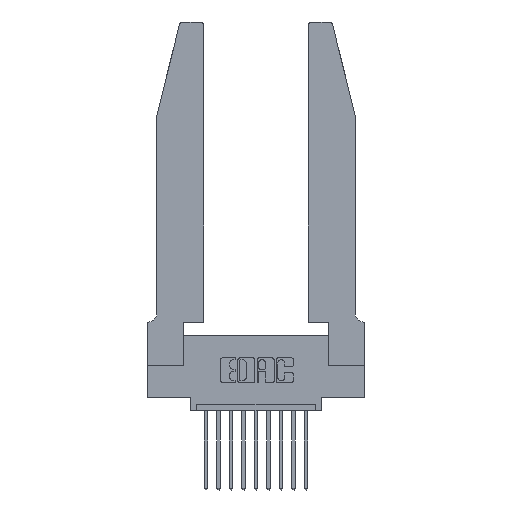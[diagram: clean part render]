
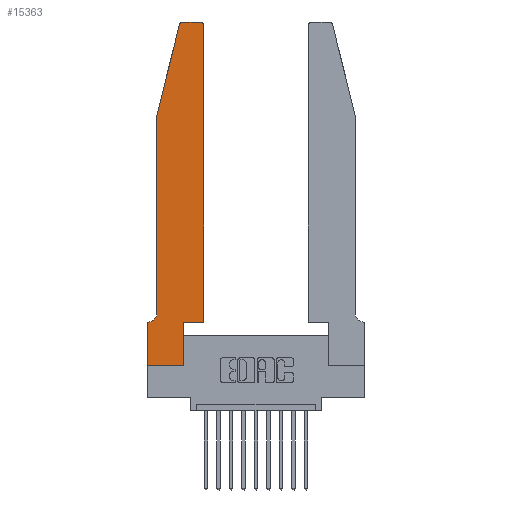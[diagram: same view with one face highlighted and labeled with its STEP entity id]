
A CAD part, top view. The second image highlights one B-rep face of the part: STEP entity #15363.
In plain terms, the highlighted planar face has unit normal (0, 0, 1).
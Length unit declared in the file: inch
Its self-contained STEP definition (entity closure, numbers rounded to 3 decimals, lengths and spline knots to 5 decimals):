
#105 = VECTOR ( 'NONE', #4149, 39.37008 ) ;
#150 = CARTESIAN_POINT ( 'NONE',  ( 0.0755, 0.35, 0.37 ) ) ;
#258 = CARTESIAN_POINT ( 'NONE',  ( 0.2865, 0.35, 0.37 ) ) ;
#534 = FACE_OUTER_BOUND ( 'NONE', #7248, .T. ) ;
#612 = AXIS2_PLACEMENT_3D ( 'NONE', #5074, #13812, #15102 ) ;
#691 = EDGE_CURVE ( 'NONE', #771, #15795, #4961, .T. ) ;
#771 = VERTEX_POINT ( 'NONE', #9427 ) ;
#926 = ORIENTED_EDGE ( 'NONE', *, *, #3100, .T. ) ;
#1084 = ORIENTED_EDGE ( 'NONE', *, *, #14314, .T. ) ;
#1206 = ORIENTED_EDGE ( 'NONE', *, *, #2494, .T. ) ;
#1215 = ORIENTED_EDGE ( 'NONE', *, *, #10130, .T. ) ;
#1451 = EDGE_CURVE ( 'NONE', #15918, #10823, #10007, .T. ) ;
#1534 = AXIS2_PLACEMENT_3D ( 'NONE', #5754, #3287, #10858 ) ;
#1617 = EDGE_CURVE ( 'NONE', #11487, #10029, #11370, .T. ) ;
#2012 = VECTOR ( 'NONE', #6888, 39.37008 ) ;
#2383 = CARTESIAN_POINT ( 'NONE',  ( 0.0055, 0.42, 0.37 ) ) ;
#2494 = EDGE_CURVE ( 'NONE', #5162, #11487, #8985, .T. ) ;
#2841 = VERTEX_POINT ( 'NONE', #3288 ) ;
#3100 = EDGE_CURVE ( 'NONE', #7993, #4041, #6681, .T. ) ;
#3287 = DIRECTION ( 'NONE',  ( 0., 0., 1. ) ) ;
#3288 = CARTESIAN_POINT ( 'NONE',  ( 0.0055, 0.35, 0.37 ) ) ;
#3401 = CARTESIAN_POINT ( 'NONE',  ( 0., 0.35, 0.37 ) ) ;
#3406 = VECTOR ( 'NONE', #9267, 39.37008 ) ;
#3431 = LINE ( 'NONE', #150, #6566 ) ;
#3547 = CARTESIAN_POINT ( 'NONE',  ( 0.4505, 0.35, 0.37 ) ) ;
#3739 = EDGE_CURVE ( 'NONE', #15795, #7993, #5899, .T. ) ;
#3815 = DIRECTION ( 'NONE',  ( 0., -1., 0. ) ) ;
#3979 = DIRECTION ( 'NONE',  ( -1., 0., 0. ) ) ;
#3980 = CARTESIAN_POINT ( 'NONE',  ( 0.0755, 2., 0.37 ) ) ;
#4041 = VERTEX_POINT ( 'NONE', #6262 ) ;
#4149 = DIRECTION ( 'NONE',  ( 0., 1., 0. ) ) ;
#4250 = CARTESIAN_POINT ( 'NONE',  ( 0.0755, 2., 0.37 ) ) ;
#4493 = ORIENTED_EDGE ( 'NONE', *, *, #1451, .T. ) ;
#4558 = CARTESIAN_POINT ( 'NONE',  ( 0.2865, 0., 0.37 ) ) ;
#4880 = DIRECTION ( 'NONE',  ( 1., 0., 0. ) ) ;
#4896 = VECTOR ( 'NONE', #8825, 39.37008 ) ;
#4961 = CIRCLE ( 'NONE', #1534, 0.03 ) ;
#5074 = CARTESIAN_POINT ( 'NONE',  ( 0., 0.35, 0.37 ) ) ;
#5162 = VERTEX_POINT ( 'NONE', #14885 ) ;
#5632 = CIRCLE ( 'NONE', #6292, 0.07 ) ;
#5754 = CARTESIAN_POINT ( 'NONE',  ( 0.284, 2.72, 0.37 ) ) ;
#5783 = EDGE_CURVE ( 'NONE', #4041, #2841, #5632, .T. ) ;
#5899 = LINE ( 'NONE', #4250, #11732 ) ;
#6000 = DIRECTION ( 'NONE',  ( 0., 0., 1. ) ) ;
#6131 = VERTEX_POINT ( 'NONE', #8067 ) ;
#6202 = LINE ( 'NONE', #3547, #14953 ) ;
#6262 = CARTESIAN_POINT ( 'NONE',  ( 0.0755, 0.42, 0.37 ) ) ;
#6292 = AXIS2_PLACEMENT_3D ( 'NONE', #2383, #14775, #15980 ) ;
#6485 = CARTESIAN_POINT ( 'NONE',  ( 0., 0., 0.37 ) ) ;
#6566 = VECTOR ( 'NONE', #3979, 39.37008 ) ;
#6681 = LINE ( 'NONE', #10018, #12892 ) ;
#6742 = ORIENTED_EDGE ( 'NONE', *, *, #6938, .T. ) ;
#6888 = DIRECTION ( 'NONE',  ( -1., 0., 0. ) ) ;
#6938 = EDGE_CURVE ( 'NONE', #2841, #12030, #3431, .T. ) ;
#7035 = ORIENTED_EDGE ( 'NONE', *, *, #3739, .T. ) ;
#7248 = EDGE_LOOP ( 'NONE', ( #1215, #13642, #7035, #926, #11999, #6742, #7647, #1206, #15122, #12852, #1084, #4493 ) ) ;
#7555 = DIRECTION ( 'NONE',  ( 0., 1., 0. ) ) ;
#7647 = ORIENTED_EDGE ( 'NONE', *, *, #16002, .T. ) ;
#7889 = VECTOR ( 'NONE', #15168, 39.37008 ) ;
#7993 = VERTEX_POINT ( 'NONE', #3980 ) ;
#8067 = CARTESIAN_POINT ( 'NONE',  ( 0.4505, 0.35, 0.37 ) ) ;
#8115 = EDGE_CURVE ( 'NONE', #10029, #6131, #14890, .T. ) ;
#8572 = CARTESIAN_POINT ( 'NONE',  ( 0.25487, 2.72718, 0.37 ) ) ;
#8825 = DIRECTION ( 'NONE',  ( 1., 0., 0. ) ) ;
#8985 = LINE ( 'NONE', #11279, #4896 ) ;
#9208 = CARTESIAN_POINT ( 'NONE',  ( 0.4505, 0.35, 0.37 ) ) ;
#9267 = DIRECTION ( 'NONE',  ( 1., 0., 0. ) ) ;
#9427 = CARTESIAN_POINT ( 'NONE',  ( 0.284, 2.75, 0.37 ) ) ;
#10007 = CIRCLE ( 'NONE', #13441, 0.03 ) ;
#10018 = CARTESIAN_POINT ( 'NONE',  ( 0.0755, 2., 0.37 ) ) ;
#10029 = VERTEX_POINT ( 'NONE', #10350 ) ;
#10130 = EDGE_CURVE ( 'NONE', #10823, #771, #12317, .T. ) ;
#10228 = CARTESIAN_POINT ( 'NONE',  ( 0.4205, 2.75, 0.37 ) ) ;
#10299 = PLANE ( 'NONE',  #612 ) ;
#10350 = CARTESIAN_POINT ( 'NONE',  ( 0.2865, 0.35, 0.37 ) ) ;
#10823 = VERTEX_POINT ( 'NONE', #10228 ) ;
#10858 = DIRECTION ( 'NONE',  ( 1., 0., 0. ) ) ;
#10880 = CARTESIAN_POINT ( 'NONE',  ( 0.4505, 2.72, 0.37 ) ) ;
#11279 = CARTESIAN_POINT ( 'NONE',  ( 0., 0., 0.37 ) ) ;
#11370 = LINE ( 'NONE', #258, #105 ) ;
#11487 = VERTEX_POINT ( 'NONE', #4558 ) ;
#11732 = VECTOR ( 'NONE', #12978, 39.37008 ) ;
#11986 = LINE ( 'NONE', #6485, #7889 ) ;
#11999 = ORIENTED_EDGE ( 'NONE', *, *, #5783, .T. ) ;
#12030 = VERTEX_POINT ( 'NONE', #3401 ) ;
#12317 = LINE ( 'NONE', #14340, #2012 ) ;
#12348 = CARTESIAN_POINT ( 'NONE',  ( 0.4205, 2.72, 0.37 ) ) ;
#12852 = ORIENTED_EDGE ( 'NONE', *, *, #8115, .T. ) ;
#12892 = VECTOR ( 'NONE', #3815, 39.37008 ) ;
#12978 = DIRECTION ( 'NONE',  ( -0.239, -0.971, 0. ) ) ;
#13441 = AXIS2_PLACEMENT_3D ( 'NONE', #12348, #6000, #4880 ) ;
#13642 = ORIENTED_EDGE ( 'NONE', *, *, #691, .T. ) ;
#13812 = DIRECTION ( 'NONE',  ( 0., 0., 1. ) ) ;
#14314 = EDGE_CURVE ( 'NONE', #6131, #15918, #6202, .T. ) ;
#14340 = CARTESIAN_POINT ( 'NONE',  ( 0.2605, 2.75, 0.37 ) ) ;
#14775 = DIRECTION ( 'NONE',  ( 0., 0., -1. ) ) ;
#14885 = CARTESIAN_POINT ( 'NONE',  ( 0., 0., 0.37 ) ) ;
#14890 = LINE ( 'NONE', #9208, #3406 ) ;
#14953 = VECTOR ( 'NONE', #7555, 39.37008 ) ;
#15102 = DIRECTION ( 'NONE',  ( 1., 0., 0. ) ) ;
#15122 = ORIENTED_EDGE ( 'NONE', *, *, #1617, .T. ) ;
#15168 = DIRECTION ( 'NONE',  ( 0., -1., 0. ) ) ;
#15363 = ADVANCED_FACE ( 'NONE', ( #534 ), #10299, .T. ) ;
#15795 = VERTEX_POINT ( 'NONE', #8572 ) ;
#15918 = VERTEX_POINT ( 'NONE', #10880 ) ;
#15980 = DIRECTION ( 'NONE',  ( -1., 0., 0. ) ) ;
#16002 = EDGE_CURVE ( 'NONE', #12030, #5162, #11986, .T. ) ;
